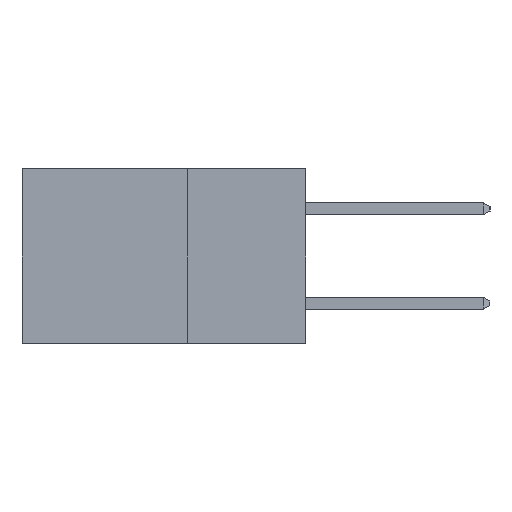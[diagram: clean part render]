
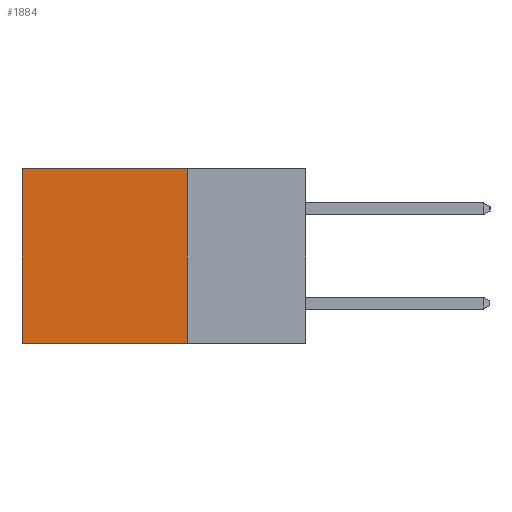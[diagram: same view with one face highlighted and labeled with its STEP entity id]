
A CAD part, left-side view. The second image highlights one B-rep face of the part: STEP entity #1884.
In plain terms, the highlighted planar face has unit normal (-1, 0, 0).
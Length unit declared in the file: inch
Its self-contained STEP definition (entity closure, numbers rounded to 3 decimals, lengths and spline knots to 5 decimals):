
#80 = DIRECTION ( 'NONE',  ( 1., 0., 0. ) ) ;
#614 = VERTEX_POINT ( 'NONE', #6692 ) ;
#725 = LINE ( 'NONE', #1745, #1632 ) ;
#806 = DIRECTION ( 'NONE',  ( 0., 0., -1. ) ) ;
#1526 = CARTESIAN_POINT ( 'NONE',  ( 0.2615, 0.25, -0.37 ) ) ;
#1632 = VECTOR ( 'NONE', #8333, 39.37008 ) ;
#1745 = CARTESIAN_POINT ( 'NONE',  ( 0.2615, 0.25, 0. ) ) ;
#1749 = ORIENTED_EDGE ( 'NONE', *, *, #11079, .F. ) ;
#1884 = ADVANCED_FACE ( 'NONE', ( #11260 ), #5463, .F. ) ;
#3258 = VERTEX_POINT ( 'NONE', #8028 ) ;
#3382 = VERTEX_POINT ( 'NONE', #4987 ) ;
#4391 = VECTOR ( 'NONE', #5263, 39.37008 ) ;
#4869 = ORIENTED_EDGE ( 'NONE', *, *, #8723, .F. ) ;
#4957 = CARTESIAN_POINT ( 'NONE',  ( 0.2615, 0.6, -0.37 ) ) ;
#4987 = CARTESIAN_POINT ( 'NONE',  ( 0.2615, 0.6, -0.37 ) ) ;
#5263 = DIRECTION ( 'NONE',  ( 0., 0., -1. ) ) ;
#5463 = PLANE ( 'NONE',  #8868 ) ;
#5597 = CARTESIAN_POINT ( 'NONE',  ( 0.2615, 0.25, -0.37 ) ) ;
#5608 = EDGE_CURVE ( 'NONE', #3258, #3382, #5761, .T. ) ;
#5720 = CARTESIAN_POINT ( 'NONE',  ( 0.2615, 0.25, -0.37 ) ) ;
#5761 = LINE ( 'NONE', #4957, #7726 ) ;
#5880 = EDGE_CURVE ( 'NONE', #614, #3258, #725, .T. ) ;
#6692 = CARTESIAN_POINT ( 'NONE',  ( 0.2615, 0.25, 0. ) ) ;
#6807 = EDGE_LOOP ( 'NONE', ( #7818, #1749, #4869, #11497 ) ) ;
#7384 = LINE ( 'NONE', #5597, #10512 ) ;
#7512 = DIRECTION ( 'NONE',  ( 0., 1., 0. ) ) ;
#7726 = VECTOR ( 'NONE', #11363, 39.37008 ) ;
#7818 = ORIENTED_EDGE ( 'NONE', *, *, #5608, .T. ) ;
#8028 = CARTESIAN_POINT ( 'NONE',  ( 0.2615, 0.6, 0. ) ) ;
#8333 = DIRECTION ( 'NONE',  ( 0., 1., 0. ) ) ;
#8723 = EDGE_CURVE ( 'NONE', #614, #11039, #9953, .T. ) ;
#8868 = AXIS2_PLACEMENT_3D ( 'NONE', #9282, #80, #806 ) ;
#9282 = CARTESIAN_POINT ( 'NONE',  ( 0.2615, 0.25, -0.37 ) ) ;
#9953 = LINE ( 'NONE', #1526, #4391 ) ;
#10512 = VECTOR ( 'NONE', #7512, 39.37008 ) ;
#11039 = VERTEX_POINT ( 'NONE', #5720 ) ;
#11079 = EDGE_CURVE ( 'NONE', #11039, #3382, #7384, .T. ) ;
#11260 = FACE_OUTER_BOUND ( 'NONE', #6807, .T. ) ;
#11363 = DIRECTION ( 'NONE',  ( 0., 0., -1. ) ) ;
#11497 = ORIENTED_EDGE ( 'NONE', *, *, #5880, .T. ) ;
